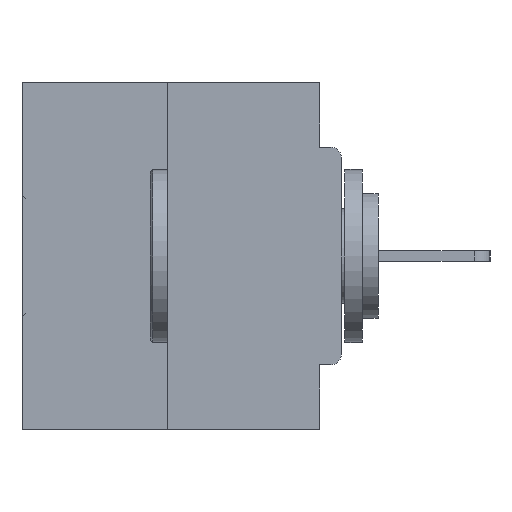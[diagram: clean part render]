
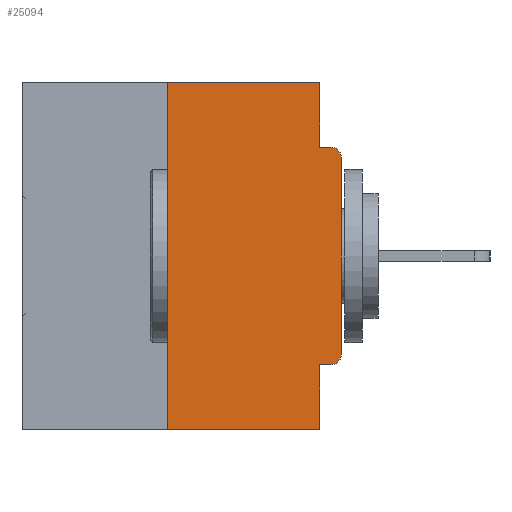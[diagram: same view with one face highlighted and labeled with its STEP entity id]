
A CAD part, left-side view. The second image highlights one B-rep face of the part: STEP entity #25094.
In plain terms, the highlighted planar face has unit normal (-1, 0, 0).
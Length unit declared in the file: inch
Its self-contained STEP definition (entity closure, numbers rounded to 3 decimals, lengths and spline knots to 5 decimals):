
#13 = DIRECTION ( 'NONE',  ( 0., -1., 0. ) ) ;
#32 = EDGE_CURVE ( 'NONE', #3318, #31308, #2403, .T. ) ;
#493 = ORIENTED_EDGE ( 'NONE', *, *, #13773, .F. ) ;
#776 = LINE ( 'NONE', #12683, #3878 ) ;
#1244 = VERTEX_POINT ( 'NONE', #29529 ) ;
#1319 = CARTESIAN_POINT ( 'NONE',  ( 0., 0., -0.3915 ) ) ;
#2403 = LINE ( 'NONE', #38114, #12392 ) ;
#2509 = VERTEX_POINT ( 'NONE', #1319 ) ;
#2826 = CARTESIAN_POINT ( 'NONE',  ( 0., 0.46, 0. ) ) ;
#2865 = LINE ( 'NONE', #20824, #7460 ) ;
#3318 = VERTEX_POINT ( 'NONE', #33980 ) ;
#3585 = CARTESIAN_POINT ( 'NONE',  ( 0., 0.25, 0. ) ) ;
#3619 = ORIENTED_EDGE ( 'NONE', *, *, #20454, .T. ) ;
#3878 = VECTOR ( 'NONE', #16206, 39.37008 ) ;
#5845 = CARTESIAN_POINT ( 'NONE',  ( 0., 0., -0.0935 ) ) ;
#6544 = VECTOR ( 'NONE', #35581, 39.37008 ) ;
#6582 = EDGE_LOOP ( 'NONE', ( #37297, #20964, #19387, #27201, #493, #9779, #34576, #3619, #26040, #28323 ) ) ;
#7460 = VECTOR ( 'NONE', #32723, 39.37008 ) ;
#8675 = CARTESIAN_POINT ( 'NONE',  ( 0., 0.25, 0. ) ) ;
#8942 = DIRECTION ( 'NONE',  ( 0., 0., -1. ) ) ;
#9207 = CARTESIAN_POINT ( 'NONE',  ( 0., 0.46, -0.5 ) ) ;
#9779 = ORIENTED_EDGE ( 'NONE', *, *, #16982, .T. ) ;
#10022 = VERTEX_POINT ( 'NONE', #8675 ) ;
#10794 = VECTOR ( 'NONE', #34997, 39.37008 ) ;
#11086 = EDGE_CURVE ( 'NONE', #15020, #10022, #22320, .T. ) ;
#11361 = DIRECTION ( 'NONE',  ( 0., 0., -1. ) ) ;
#12368 = EDGE_CURVE ( 'NONE', #10022, #36159, #34228, .T. ) ;
#12392 = VECTOR ( 'NONE', #11361, 39.37008 ) ;
#12585 = CIRCLE ( 'NONE', #22572, 0.015 ) ;
#12683 = CARTESIAN_POINT ( 'NONE',  ( 0., 0., 0. ) ) ;
#13773 = EDGE_CURVE ( 'NONE', #1244, #3318, #2865, .T. ) ;
#14541 = PLANE ( 'NONE',  #22156 ) ;
#14542 = EDGE_CURVE ( 'NONE', #37158, #20509, #30040, .T. ) ;
#15020 = VERTEX_POINT ( 'NONE', #29406 ) ;
#16206 = DIRECTION ( 'NONE',  ( 0., 0., 1. ) ) ;
#16826 = EDGE_CURVE ( 'NONE', #36159, #37158, #19376, .T. ) ;
#16982 = EDGE_CURVE ( 'NONE', #1244, #2509, #36967, .T. ) ;
#17932 = DIRECTION ( 'NONE',  ( -1., 0., 0. ) ) ;
#18787 = DIRECTION ( 'NONE',  ( 0., 0., 1. ) ) ;
#18796 = DIRECTION ( 'NONE',  ( 0., -1., 0. ) ) ;
#19376 = LINE ( 'NONE', #34620, #10794 ) ;
#19387 = ORIENTED_EDGE ( 'NONE', *, *, #29837, .T. ) ;
#19892 = VECTOR ( 'NONE', #18796, 39.37008 ) ;
#20454 = EDGE_CURVE ( 'NONE', #34979, #20509, #12585, .T. ) ;
#20509 = VERTEX_POINT ( 'NONE', #35690 ) ;
#20824 = CARTESIAN_POINT ( 'NONE',  ( 0., 0., -0.4065 ) ) ;
#20964 = ORIENTED_EDGE ( 'NONE', *, *, #11086, .F. ) ;
#22156 = AXIS2_PLACEMENT_3D ( 'NONE', #2826, #23729, #35625 ) ;
#22196 = VECTOR ( 'NONE', #18787, 39.37008 ) ;
#22320 = LINE ( 'NONE', #3585, #22196 ) ;
#22572 = AXIS2_PLACEMENT_3D ( 'NONE', #30207, #17932, #8942 ) ;
#22715 = EDGE_CURVE ( 'NONE', #2509, #34979, #776, .T. ) ;
#23276 = AXIS2_PLACEMENT_3D ( 'NONE', #32649, #26406, #23876 ) ;
#23683 = LINE ( 'NONE', #9207, #6544 ) ;
#23729 = DIRECTION ( 'NONE',  ( 1., 0., 0. ) ) ;
#23876 = DIRECTION ( 'NONE',  ( 0., 0., -1. ) ) ;
#24412 = CARTESIAN_POINT ( 'NONE',  ( 0., 0., -0.1085 ) ) ;
#24912 = CARTESIAN_POINT ( 'NONE',  ( 0., 0.031, -0.0935 ) ) ;
#25094 = ADVANCED_FACE ( 'NONE', ( #29361 ), #14541, .F. ) ;
#26040 = ORIENTED_EDGE ( 'NONE', *, *, #14542, .F. ) ;
#26406 = DIRECTION ( 'NONE',  ( -1., 0., 0. ) ) ;
#27201 = ORIENTED_EDGE ( 'NONE', *, *, #32, .F. ) ;
#27522 = CARTESIAN_POINT ( 'NONE',  ( 0., 0.031, 0. ) ) ;
#28305 = CARTESIAN_POINT ( 'NONE',  ( 0., 0.031, -0.5 ) ) ;
#28323 = ORIENTED_EDGE ( 'NONE', *, *, #16826, .F. ) ;
#29361 = FACE_OUTER_BOUND ( 'NONE', #6582, .T. ) ;
#29406 = CARTESIAN_POINT ( 'NONE',  ( 0., 0.25, -0.5 ) ) ;
#29529 = CARTESIAN_POINT ( 'NONE',  ( 0., 0.015, -0.4065 ) ) ;
#29837 = EDGE_CURVE ( 'NONE', #15020, #31308, #23683, .T. ) ;
#30040 = LINE ( 'NONE', #5845, #33271 ) ;
#30207 = CARTESIAN_POINT ( 'NONE',  ( 0., 0.015, -0.1085 ) ) ;
#31097 = CARTESIAN_POINT ( 'NONE',  ( 0., 0.46, 0. ) ) ;
#31308 = VERTEX_POINT ( 'NONE', #28305 ) ;
#32649 = CARTESIAN_POINT ( 'NONE',  ( 0., 0.015, -0.3915 ) ) ;
#32723 = DIRECTION ( 'NONE',  ( 0., 1., 0. ) ) ;
#33271 = VECTOR ( 'NONE', #13, 39.37008 ) ;
#33980 = CARTESIAN_POINT ( 'NONE',  ( 0., 0.031, -0.4065 ) ) ;
#34228 = LINE ( 'NONE', #31097, #19892 ) ;
#34576 = ORIENTED_EDGE ( 'NONE', *, *, #22715, .T. ) ;
#34620 = CARTESIAN_POINT ( 'NONE',  ( 0., 0.031, 0. ) ) ;
#34979 = VERTEX_POINT ( 'NONE', #24412 ) ;
#34997 = DIRECTION ( 'NONE',  ( 0., 0., -1. ) ) ;
#35581 = DIRECTION ( 'NONE',  ( 0., -1., 0. ) ) ;
#35625 = DIRECTION ( 'NONE',  ( 0., 0., -1. ) ) ;
#35690 = CARTESIAN_POINT ( 'NONE',  ( 0., 0.015, -0.0935 ) ) ;
#36159 = VERTEX_POINT ( 'NONE', #27522 ) ;
#36967 = CIRCLE ( 'NONE', #23276, 0.015 ) ;
#37158 = VERTEX_POINT ( 'NONE', #24912 ) ;
#37297 = ORIENTED_EDGE ( 'NONE', *, *, #12368, .F. ) ;
#38114 = CARTESIAN_POINT ( 'NONE',  ( 0., 0.031, -0.5 ) ) ;
